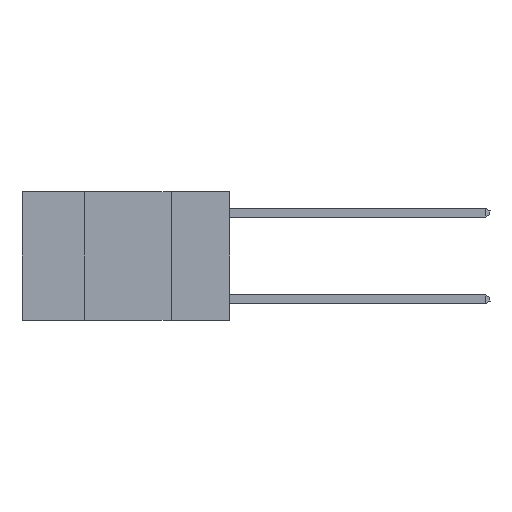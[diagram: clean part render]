
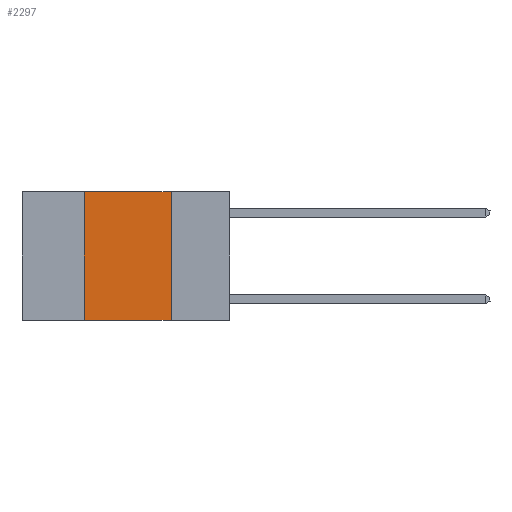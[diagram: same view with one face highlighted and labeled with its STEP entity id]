
A CAD part, left-side view. The second image highlights one B-rep face of the part: STEP entity #2297.
In plain terms, the highlighted planar face has unit normal (-1, 0, 0).
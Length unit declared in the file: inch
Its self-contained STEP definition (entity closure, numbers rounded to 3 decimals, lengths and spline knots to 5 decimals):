
#287 = CARTESIAN_POINT ( 'NONE',  ( 0., 0.17, 0. ) ) ;
#295 = VECTOR ( 'NONE', #8001, 39.37008 ) ;
#718 = DIRECTION ( 'NONE',  ( 1., 0., 0. ) ) ;
#765 = CARTESIAN_POINT ( 'NONE',  ( 0., 0.17, 0. ) ) ;
#1236 = DIRECTION ( 'NONE',  ( 0., 0., -1. ) ) ;
#1427 = CARTESIAN_POINT ( 'NONE',  ( 0., 0.17, -0.37 ) ) ;
#1598 = DIRECTION ( 'NONE',  ( 0., 0., 1. ) ) ;
#2174 = VECTOR ( 'NONE', #10983, 39.37008 ) ;
#2297 = ADVANCED_FACE ( 'NONE', ( #6435 ), #10908, .F. ) ;
#2619 = CARTESIAN_POINT ( 'NONE',  ( 0., 0.6, -0.37 ) ) ;
#2864 = EDGE_CURVE ( 'NONE', #7660, #8969, #5840, .T. ) ;
#3061 = EDGE_LOOP ( 'NONE', ( #5747, #8804, #9095, #4722 ) ) ;
#3117 = LINE ( 'NONE', #7178, #5607 ) ;
#3837 = CARTESIAN_POINT ( 'NONE',  ( 0., 0.42, 0. ) ) ;
#4565 = AXIS2_PLACEMENT_3D ( 'NONE', #11845, #718, #7242 ) ;
#4722 = ORIENTED_EDGE ( 'NONE', *, *, #4986, .T. ) ;
#4986 = EDGE_CURVE ( 'NONE', #5563, #10667, #9301, .T. ) ;
#5563 = VERTEX_POINT ( 'NONE', #7222 ) ;
#5607 = VECTOR ( 'NONE', #1598, 39.37008 ) ;
#5747 = ORIENTED_EDGE ( 'NONE', *, *, #8659, .F. ) ;
#5840 = LINE ( 'NONE', #6125, #295 ) ;
#6125 = CARTESIAN_POINT ( 'NONE',  ( 0., 0.6, 0. ) ) ;
#6280 = LINE ( 'NONE', #287, #10603 ) ;
#6435 = FACE_OUTER_BOUND ( 'NONE', #3061, .T. ) ;
#7178 = CARTESIAN_POINT ( 'NONE',  ( 0., 0.42, 0. ) ) ;
#7222 = CARTESIAN_POINT ( 'NONE',  ( 0., 0.42, -0.37 ) ) ;
#7242 = DIRECTION ( 'NONE',  ( 0., 0., -1. ) ) ;
#7406 = EDGE_CURVE ( 'NONE', #5563, #7660, #3117, .T. ) ;
#7660 = VERTEX_POINT ( 'NONE', #3837 ) ;
#8001 = DIRECTION ( 'NONE',  ( 0., -1., 0. ) ) ;
#8659 = EDGE_CURVE ( 'NONE', #8969, #10667, #6280, .T. ) ;
#8804 = ORIENTED_EDGE ( 'NONE', *, *, #2864, .F. ) ;
#8969 = VERTEX_POINT ( 'NONE', #765 ) ;
#9095 = ORIENTED_EDGE ( 'NONE', *, *, #7406, .F. ) ;
#9301 = LINE ( 'NONE', #2619, #2174 ) ;
#10603 = VECTOR ( 'NONE', #1236, 39.37008 ) ;
#10667 = VERTEX_POINT ( 'NONE', #1427 ) ;
#10908 = PLANE ( 'NONE',  #4565 ) ;
#10983 = DIRECTION ( 'NONE',  ( 0., -1., 0. ) ) ;
#11845 = CARTESIAN_POINT ( 'NONE',  ( 0., 0.6, 0. ) ) ;
